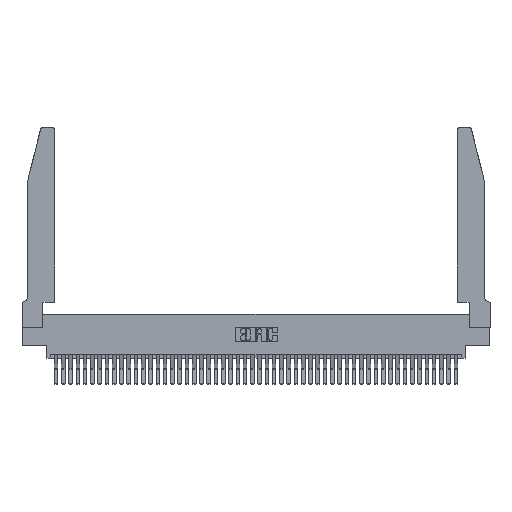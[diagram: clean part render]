
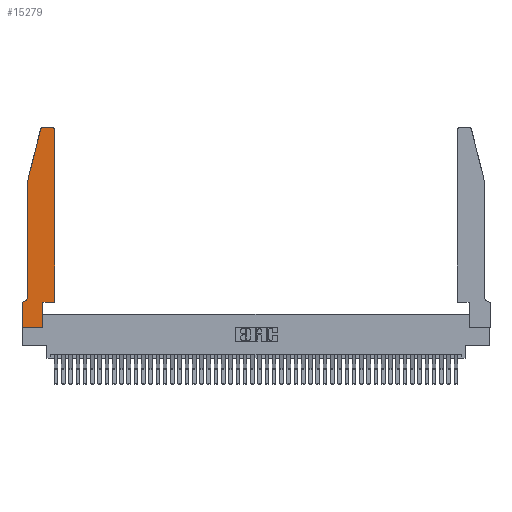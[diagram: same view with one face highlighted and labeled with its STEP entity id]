
A CAD part, top view. The second image highlights one B-rep face of the part: STEP entity #15279.
In plain terms, the highlighted planar face has unit normal (0, 0, 1).
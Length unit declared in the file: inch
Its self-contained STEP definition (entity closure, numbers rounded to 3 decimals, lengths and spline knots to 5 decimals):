
#124 = VECTOR ( 'NONE', #6725, 39.37008 ) ;
#393 = EDGE_CURVE ( 'NONE', #40542, #21041, #15526, .T. ) ;
#1397 = VERTEX_POINT ( 'NONE', #13483 ) ;
#2510 = EDGE_CURVE ( 'NONE', #10419, #2663, #41785, .T. ) ;
#2663 = VERTEX_POINT ( 'NONE', #42467 ) ;
#3539 = AXIS2_PLACEMENT_3D ( 'NONE', #5912, #34935, #35727 ) ;
#4077 = ORIENTED_EDGE ( 'NONE', *, *, #8106, .T. ) ;
#4586 = EDGE_CURVE ( 'NONE', #21041, #1397, #19382, .T. ) ;
#4891 = CARTESIAN_POINT ( 'NONE',  ( 0.25487, 2.72718, 0.37 ) ) ;
#5341 = VERTEX_POINT ( 'NONE', #44386 ) ;
#5378 = DIRECTION ( 'NONE',  ( 1., 0., 0. ) ) ;
#5441 = AXIS2_PLACEMENT_3D ( 'NONE', #13650, #6811, #17272 ) ;
#5875 = LINE ( 'NONE', #47044, #26232 ) ;
#5881 = DIRECTION ( 'NONE',  ( 0., 0., 1. ) ) ;
#5912 = CARTESIAN_POINT ( 'NONE',  ( 0.4205, 2.72, 0.37 ) ) ;
#5986 = DIRECTION ( 'NONE',  ( 0., 1., 0. ) ) ;
#6431 = VECTOR ( 'NONE', #14494, 39.37008 ) ;
#6725 = DIRECTION ( 'NONE',  ( -1., 0., 0. ) ) ;
#6811 = DIRECTION ( 'NONE',  ( 0., 0., -1. ) ) ;
#7722 = AXIS2_PLACEMENT_3D ( 'NONE', #34561, #5881, #5378 ) ;
#8106 = EDGE_CURVE ( 'NONE', #17133, #40542, #42428, .T. ) ;
#9448 = PLANE ( 'NONE',  #16415 ) ;
#10419 = VERTEX_POINT ( 'NONE', #11286 ) ;
#11286 = CARTESIAN_POINT ( 'NONE',  ( 0.2865, 0., 0.37 ) ) ;
#11907 = DIRECTION ( 'NONE',  ( 0., 1., 0. ) ) ;
#12127 = EDGE_LOOP ( 'NONE', ( #46336, #14570, #37960, #41970, #21716, #28138, #36635, #23978, #23414, #14165, #4077, #41536 ) ) ;
#13010 = LINE ( 'NONE', #45352, #42559 ) ;
#13128 = CARTESIAN_POINT ( 'NONE',  ( 0., 0.35, 0.37 ) ) ;
#13483 = CARTESIAN_POINT ( 'NONE',  ( 0.284, 2.75, 0.37 ) ) ;
#13650 = CARTESIAN_POINT ( 'NONE',  ( 0.0055, 0.42, 0.37 ) ) ;
#14165 = ORIENTED_EDGE ( 'NONE', *, *, #18336, .T. ) ;
#14494 = DIRECTION ( 'NONE',  ( 0., -1., 0. ) ) ;
#14570 = ORIENTED_EDGE ( 'NONE', *, *, #16078, .T. ) ;
#15279 = ADVANCED_FACE ( 'NONE', ( #30269 ), #9448, .T. ) ;
#15526 = CIRCLE ( 'NONE', #3539, 0.03 ) ;
#16078 = EDGE_CURVE ( 'NONE', #1397, #18877, #31921, .T. ) ;
#16290 = DIRECTION ( 'NONE',  ( 1., 0., 0. ) ) ;
#16415 = AXIS2_PLACEMENT_3D ( 'NONE', #13128, #20357, #16290 ) ;
#16548 = CARTESIAN_POINT ( 'NONE',  ( 0.4205, 2.75, 0.37 ) ) ;
#16622 = CARTESIAN_POINT ( 'NONE',  ( 0.0755, 2., 0.37 ) ) ;
#16686 = VECTOR ( 'NONE', #30532, 39.37008 ) ;
#16820 = VERTEX_POINT ( 'NONE', #26349 ) ;
#17133 = VERTEX_POINT ( 'NONE', #24576 ) ;
#17272 = DIRECTION ( 'NONE',  ( -1., 0., 0. ) ) ;
#18297 = VERTEX_POINT ( 'NONE', #35868 ) ;
#18336 = EDGE_CURVE ( 'NONE', #2663, #17133, #45424, .T. ) ;
#18877 = VERTEX_POINT ( 'NONE', #4891 ) ;
#19382 = LINE ( 'NONE', #20807, #124 ) ;
#19737 = DIRECTION ( 'NONE',  ( -0.239, -0.971, 0. ) ) ;
#20357 = DIRECTION ( 'NONE',  ( 0., 0., 1. ) ) ;
#20807 = CARTESIAN_POINT ( 'NONE',  ( 0.2605, 2.75, 0.37 ) ) ;
#21041 = VERTEX_POINT ( 'NONE', #16548 ) ;
#21716 = ORIENTED_EDGE ( 'NONE', *, *, #33218, .T. ) ;
#23414 = ORIENTED_EDGE ( 'NONE', *, *, #2510, .T. ) ;
#23977 = LINE ( 'NONE', #28904, #6431 ) ;
#23978 = ORIENTED_EDGE ( 'NONE', *, *, #43604, .T. ) ;
#24576 = CARTESIAN_POINT ( 'NONE',  ( 0.4505, 0.35, 0.37 ) ) ;
#24789 = CARTESIAN_POINT ( 'NONE',  ( 0.0055, 0.35, 0.37 ) ) ;
#25079 = CARTESIAN_POINT ( 'NONE',  ( 0.0755, 2., 0.37 ) ) ;
#26232 = VECTOR ( 'NONE', #46882, 39.37008 ) ;
#26349 = CARTESIAN_POINT ( 'NONE',  ( 0.0755, 0.42, 0.37 ) ) ;
#26573 = CARTESIAN_POINT ( 'NONE',  ( 0., 0., 0.37 ) ) ;
#28138 = ORIENTED_EDGE ( 'NONE', *, *, #39170, .T. ) ;
#28904 = CARTESIAN_POINT ( 'NONE',  ( 0.0755, 2., 0.37 ) ) ;
#29124 = EDGE_CURVE ( 'NONE', #18297, #5341, #36555, .T. ) ;
#29728 = VECTOR ( 'NONE', #19737, 39.37008 ) ;
#29798 = VECTOR ( 'NONE', #11907, 39.37008 ) ;
#29991 = VERTEX_POINT ( 'NONE', #24789 ) ;
#30269 = FACE_OUTER_BOUND ( 'NONE', #12127, .T. ) ;
#30532 = DIRECTION ( 'NONE',  ( 0., -1., 0. ) ) ;
#31613 = CARTESIAN_POINT ( 'NONE',  ( 0.4505, 0.35, 0.37 ) ) ;
#31921 = CIRCLE ( 'NONE', #7722, 0.03 ) ;
#33218 = EDGE_CURVE ( 'NONE', #16820, #29991, #33878, .T. ) ;
#33456 = CARTESIAN_POINT ( 'NONE',  ( 0.4505, 0.35, 0.37 ) ) ;
#33878 = CIRCLE ( 'NONE', #5441, 0.07 ) ;
#34530 = VERTEX_POINT ( 'NONE', #25079 ) ;
#34561 = CARTESIAN_POINT ( 'NONE',  ( 0.284, 2.72, 0.37 ) ) ;
#34935 = DIRECTION ( 'NONE',  ( 0., 0., 1. ) ) ;
#35172 = CARTESIAN_POINT ( 'NONE',  ( 0.2865, 0.35, 0.37 ) ) ;
#35727 = DIRECTION ( 'NONE',  ( 1., 0., 0. ) ) ;
#35868 = CARTESIAN_POINT ( 'NONE',  ( 0., 0.35, 0.37 ) ) ;
#36222 = DIRECTION ( 'NONE',  ( 1., 0., 0. ) ) ;
#36555 = LINE ( 'NONE', #26573, #16686 ) ;
#36635 = ORIENTED_EDGE ( 'NONE', *, *, #29124, .T. ) ;
#37178 = VECTOR ( 'NONE', #5986, 39.37008 ) ;
#37705 = DIRECTION ( 'NONE',  ( -1., 0., 0. ) ) ;
#37960 = ORIENTED_EDGE ( 'NONE', *, *, #42734, .T. ) ;
#38856 = LINE ( 'NONE', #16622, #29728 ) ;
#39170 = EDGE_CURVE ( 'NONE', #29991, #18297, #13010, .T. ) ;
#40542 = VERTEX_POINT ( 'NONE', #42246 ) ;
#41446 = VECTOR ( 'NONE', #36222, 39.37008 ) ;
#41536 = ORIENTED_EDGE ( 'NONE', *, *, #393, .T. ) ;
#41785 = LINE ( 'NONE', #35172, #37178 ) ;
#41970 = ORIENTED_EDGE ( 'NONE', *, *, #43593, .T. ) ;
#42246 = CARTESIAN_POINT ( 'NONE',  ( 0.4505, 2.72, 0.37 ) ) ;
#42428 = LINE ( 'NONE', #33456, #29798 ) ;
#42467 = CARTESIAN_POINT ( 'NONE',  ( 0.2865, 0.35, 0.37 ) ) ;
#42559 = VECTOR ( 'NONE', #37705, 39.37008 ) ;
#42734 = EDGE_CURVE ( 'NONE', #18877, #34530, #38856, .T. ) ;
#43593 = EDGE_CURVE ( 'NONE', #34530, #16820, #23977, .T. ) ;
#43604 = EDGE_CURVE ( 'NONE', #5341, #10419, #5875, .T. ) ;
#44386 = CARTESIAN_POINT ( 'NONE',  ( 0., 0., 0.37 ) ) ;
#45352 = CARTESIAN_POINT ( 'NONE',  ( 0.0755, 0.35, 0.37 ) ) ;
#45424 = LINE ( 'NONE', #31613, #41446 ) ;
#46336 = ORIENTED_EDGE ( 'NONE', *, *, #4586, .T. ) ;
#46882 = DIRECTION ( 'NONE',  ( 1., 0., 0. ) ) ;
#47044 = CARTESIAN_POINT ( 'NONE',  ( 0., 0., 0.37 ) ) ;
